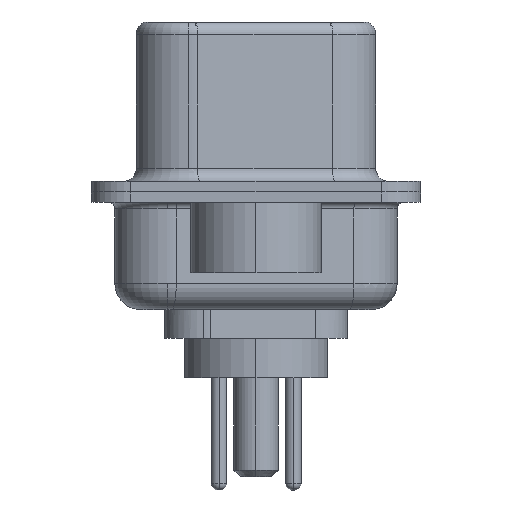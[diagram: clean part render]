
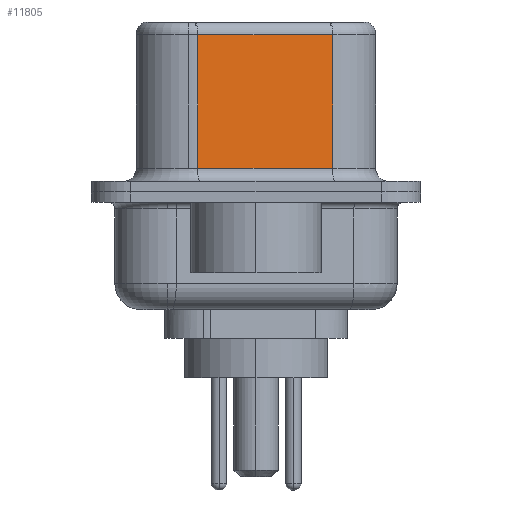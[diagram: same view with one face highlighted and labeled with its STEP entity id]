
A CAD part, left-side view. The second image highlights one B-rep face of the part: STEP entity #11805.
In plain terms, the highlighted planar face has unit normal (-0.985, -0.174, 0).
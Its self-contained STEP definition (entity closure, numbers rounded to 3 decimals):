
#322 = VERTEX_POINT ( 'NONE', #4200 ) ;
#391 = EDGE_CURVE ( 'NONE', #322, #18546, #6798, .T. ) ;
#982 = CARTESIAN_POINT ( 'NONE',  ( 4.58, -2.927, 6.02 ) ) ;
#2271 = VECTOR ( 'NONE', #13347, 1000. ) ;
#3930 = CARTESIAN_POINT ( 'NONE',  ( 4.58, -2.927, 6.52 ) ) ;
#4200 = CARTESIAN_POINT ( 'NONE',  ( 3.67, 2.233, 6.02 ) ) ;
#4919 = CARTESIAN_POINT ( 'NONE',  ( 3.67, 2.233, 0.9 ) ) ;
#4999 = CARTESIAN_POINT ( 'NONE',  ( 4.58, -2.927, 6.02 ) ) ;
#5097 = ORIENTED_EDGE ( 'NONE', *, *, #391, .T. ) ;
#5764 = ORIENTED_EDGE ( 'NONE', *, *, #9789, .F. ) ;
#5774 = LINE ( 'NONE', #4999, #19101 ) ;
#6220 = ORIENTED_EDGE ( 'NONE', *, *, #19697, .T. ) ;
#6798 = LINE ( 'NONE', #13461, #11411 ) ;
#7166 = LINE ( 'NONE', #11628, #2271 ) ;
#9036 = CARTESIAN_POINT ( 'NONE',  ( 4.58, -2.927, 6.52 ) ) ;
#9592 = FACE_OUTER_BOUND ( 'NONE', #19106, .T. ) ;
#9789 = EDGE_CURVE ( 'NONE', #13897, #17883, #21043, .T. ) ;
#10243 = ORIENTED_EDGE ( 'NONE', *, *, #16479, .T. ) ;
#10701 = DIRECTION ( 'NONE',  ( -0.174, 0.985, 0. ) ) ;
#11411 = VECTOR ( 'NONE', #17434, 1000. ) ;
#11585 = DIRECTION ( 'NONE',  ( 0., 0., -1. ) ) ;
#11628 = CARTESIAN_POINT ( 'NONE',  ( 4.58, -2.927, 0.9 ) ) ;
#11805 = ADVANCED_FACE ( 'NONE', ( #9592 ), #18935, .F. ) ;
#11886 = VECTOR ( 'NONE', #11585, 1000. ) ;
#13347 = DIRECTION ( 'NONE',  ( 0.174, -0.985, 0. ) ) ;
#13373 = AXIS2_PLACEMENT_3D ( 'NONE', #3930, #20523, #10701 ) ;
#13461 = CARTESIAN_POINT ( 'NONE',  ( 3.67, 2.233, 6.52 ) ) ;
#13897 = VERTEX_POINT ( 'NONE', #982 ) ;
#16479 = EDGE_CURVE ( 'NONE', #13897, #322, #5774, .T. ) ;
#16488 = CARTESIAN_POINT ( 'NONE',  ( 4.58, -2.927, 0.9 ) ) ;
#17434 = DIRECTION ( 'NONE',  ( 0., 0., -1. ) ) ;
#17883 = VERTEX_POINT ( 'NONE', #16488 ) ;
#18421 = DIRECTION ( 'NONE',  ( -0.174, 0.985, 0. ) ) ;
#18546 = VERTEX_POINT ( 'NONE', #4919 ) ;
#18935 = PLANE ( 'NONE',  #13373 ) ;
#19101 = VECTOR ( 'NONE', #18421, 1000. ) ;
#19106 = EDGE_LOOP ( 'NONE', ( #5764, #10243, #5097, #6220 ) ) ;
#19697 = EDGE_CURVE ( 'NONE', #18546, #17883, #7166, .T. ) ;
#20523 = DIRECTION ( 'NONE',  ( 0.985, 0.174, 0. ) ) ;
#21043 = LINE ( 'NONE', #9036, #11886 ) ;
